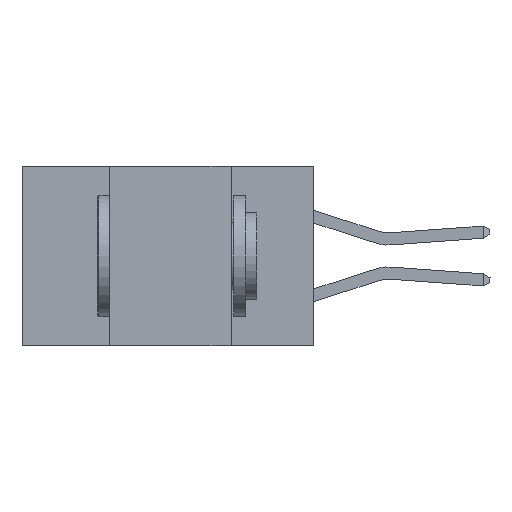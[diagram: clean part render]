
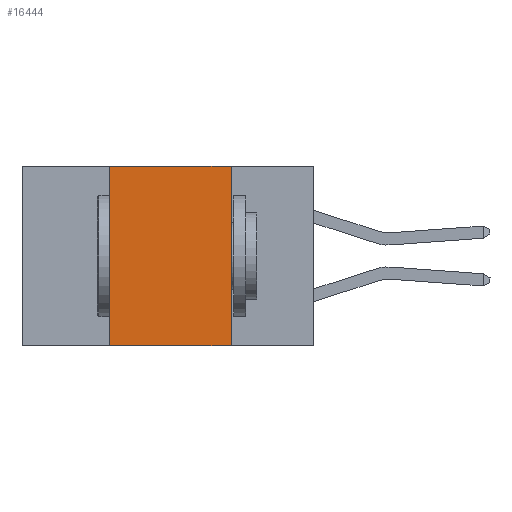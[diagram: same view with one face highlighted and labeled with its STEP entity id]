
A CAD part, left-side view. The second image highlights one B-rep face of the part: STEP entity #16444.
In plain terms, the highlighted planar face has unit normal (-1, 0, 0).
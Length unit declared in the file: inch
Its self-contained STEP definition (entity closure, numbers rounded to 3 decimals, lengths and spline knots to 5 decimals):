
#466 = CARTESIAN_POINT ( 'NONE',  ( 0., 0.17, 0. ) ) ;
#1095 = LINE ( 'NONE', #15754, #4171 ) ;
#2121 = EDGE_CURVE ( 'NONE', #12249, #13077, #14816, .T. ) ;
#2128 = LINE ( 'NONE', #4871, #8530 ) ;
#2131 = CARTESIAN_POINT ( 'NONE',  ( 0., 0.17, -0.37 ) ) ;
#2154 = CARTESIAN_POINT ( 'NONE',  ( 0., 0.42, 0. ) ) ;
#2210 = DIRECTION ( 'NONE',  ( 0., 0., 1. ) ) ;
#2989 = EDGE_CURVE ( 'NONE', #7285, #4885, #14352, .T. ) ;
#3659 = AXIS2_PLACEMENT_3D ( 'NONE', #7795, #12998, #5296 ) ;
#4171 = VECTOR ( 'NONE', #15655, 39.37008 ) ;
#4715 = EDGE_CURVE ( 'NONE', #7285, #13077, #1095, .T. ) ;
#4871 = CARTESIAN_POINT ( 'NONE',  ( 0., 0.6, 0. ) ) ;
#4885 = VERTEX_POINT ( 'NONE', #13127 ) ;
#5116 = EDGE_LOOP ( 'NONE', ( #6731, #12530, #5813, #13268 ) ) ;
#5296 = DIRECTION ( 'NONE',  ( 0., 0., -1. ) ) ;
#5813 = ORIENTED_EDGE ( 'NONE', *, *, #2989, .F. ) ;
#6146 = DIRECTION ( 'NONE',  ( 0., -1., 0. ) ) ;
#6731 = ORIENTED_EDGE ( 'NONE', *, *, #2121, .F. ) ;
#7285 = VERTEX_POINT ( 'NONE', #11495 ) ;
#7795 = CARTESIAN_POINT ( 'NONE',  ( 0., 0.6, 0. ) ) ;
#7868 = VECTOR ( 'NONE', #10906, 39.37008 ) ;
#8530 = VECTOR ( 'NONE', #6146, 39.37008 ) ;
#8618 = VECTOR ( 'NONE', #2210, 39.37008 ) ;
#9673 = FACE_OUTER_BOUND ( 'NONE', #5116, .T. ) ;
#10906 = DIRECTION ( 'NONE',  ( 0., 0., -1. ) ) ;
#11495 = CARTESIAN_POINT ( 'NONE',  ( 0., 0.42, -0.37 ) ) ;
#11676 = PLANE ( 'NONE',  #3659 ) ;
#12249 = VERTEX_POINT ( 'NONE', #466 ) ;
#12530 = ORIENTED_EDGE ( 'NONE', *, *, #14456, .F. ) ;
#12998 = DIRECTION ( 'NONE',  ( 1., 0., 0. ) ) ;
#13077 = VERTEX_POINT ( 'NONE', #2131 ) ;
#13127 = CARTESIAN_POINT ( 'NONE',  ( 0., 0.42, 0. ) ) ;
#13268 = ORIENTED_EDGE ( 'NONE', *, *, #4715, .T. ) ;
#14352 = LINE ( 'NONE', #2154, #8618 ) ;
#14456 = EDGE_CURVE ( 'NONE', #4885, #12249, #2128, .T. ) ;
#14816 = LINE ( 'NONE', #16098, #7868 ) ;
#15655 = DIRECTION ( 'NONE',  ( 0., -1., 0. ) ) ;
#15754 = CARTESIAN_POINT ( 'NONE',  ( 0., 0.6, -0.37 ) ) ;
#16098 = CARTESIAN_POINT ( 'NONE',  ( 0., 0.17, 0. ) ) ;
#16444 = ADVANCED_FACE ( 'NONE', ( #9673 ), #11676, .F. ) ;
